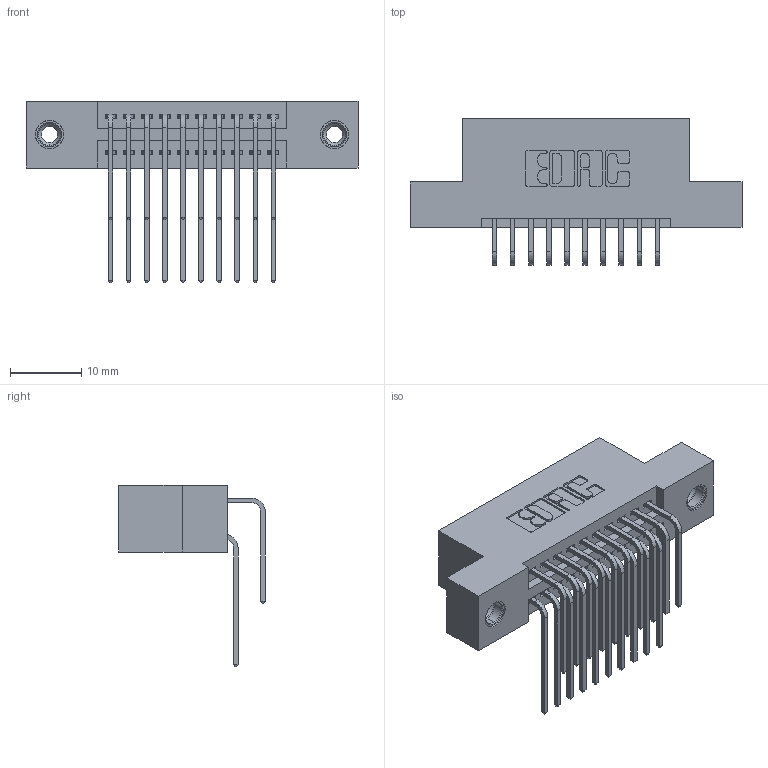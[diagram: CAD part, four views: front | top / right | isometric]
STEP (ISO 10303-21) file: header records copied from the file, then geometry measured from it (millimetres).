
FILE_DESCRIPTION (( 'STEP AP203' ), '1' );
FILE_NAME ('395-020-559-208.STEP', '2019-10-15T22:07:55', ( '' ), ( '' ), 'SwSTEP 2.0', 'SolidWorks 2016', '' );
FILE_SCHEMA (( 'CONFIG_CONTROL_DESIGN' ));
Length unit declared in the file: inch
Products named in the file (5): 345 Part_Flush Mounting Lugs - 0.156 Dia-TI; 345-292-001_558 559 Tail - 1; 345-292-001_559 Tail - 2; 345-250-001_345-250-003-102; 395-020-559-208
Assembly tree (23 placements, depth 2):
  395-020-559-208
    345 Part_Flush Mounting Lugs - 0.156 Dia-TI
    345-292-001_558 559 Tail - 1  x10
    345-292-001_559 Tail - 2  x10
    345-250-001_345-250-003-102  x2
Bounding box: 46.61 x 20.56 x 25.53 mm (x, y, z)
Volume: 4339.5 mm3; surface area: 6350.7 mm2
Topology: 23 solids, 23 shells, 1226 faces, 3577 edges, 2350 vertices
Faces by surface type: plane 812, cylinder 398, cone 12, torus 4
Entity records: 14992 total; most frequent: CARTESIAN_POINT 2570, ORIENTED_EDGE 2446, DIRECTION 2305, EDGE_CURVE 1223, LINE 991, VECTOR 991, VERTEX_POINT 808, AXIS2_PLACEMENT_3D 657
